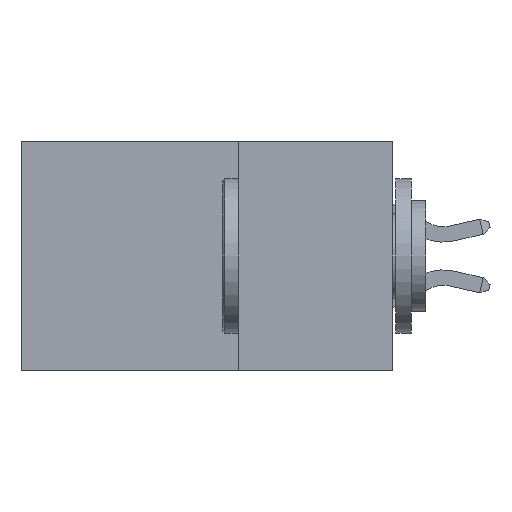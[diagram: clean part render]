
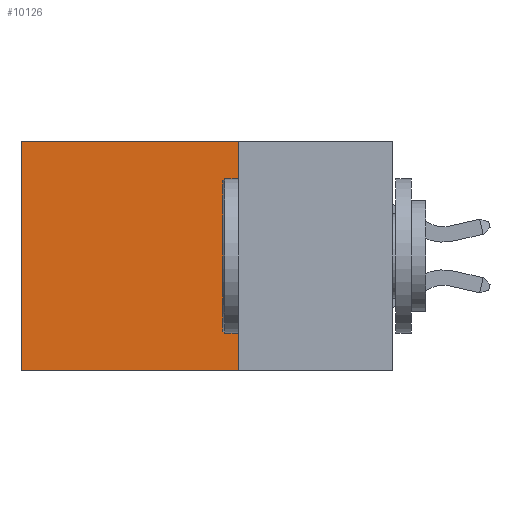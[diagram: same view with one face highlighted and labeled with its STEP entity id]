
A CAD part, left-side view. The second image highlights one B-rep face of the part: STEP entity #10126.
In plain terms, the highlighted planar face has unit normal (-1, 0, 0).
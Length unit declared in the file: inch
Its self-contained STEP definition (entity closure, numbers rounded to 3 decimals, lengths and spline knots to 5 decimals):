
#31 = VERTEX_POINT ( 'NONE', #9871 ) ;
#461 = EDGE_CURVE ( 'NONE', #31, #5469, #11803, .T. ) ;
#517 = CARTESIAN_POINT ( 'NONE',  ( 0.2875, 0.6, 0. ) ) ;
#1117 = LINE ( 'NONE', #2367, #7731 ) ;
#1857 = ORIENTED_EDGE ( 'NONE', *, *, #10371, .F. ) ;
#2362 = VECTOR ( 'NONE', #10039, 39.37008 ) ;
#2367 = CARTESIAN_POINT ( 'NONE',  ( 0.2875, 0.6, 0. ) ) ;
#2748 = ORIENTED_EDGE ( 'NONE', *, *, #461, .T. ) ;
#2933 = CARTESIAN_POINT ( 'NONE',  ( 0.2875, 0.25, -0.37 ) ) ;
#4209 = ORIENTED_EDGE ( 'NONE', *, *, #10594, .T. ) ;
#4328 = DIRECTION ( 'NONE',  ( 0., 0., -1. ) ) ;
#5469 = VERTEX_POINT ( 'NONE', #517 ) ;
#7024 = VECTOR ( 'NONE', #10593, 39.37008 ) ;
#7731 = VECTOR ( 'NONE', #4328, 39.37008 ) ;
#8003 = VERTEX_POINT ( 'NONE', #11242 ) ;
#8195 = CARTESIAN_POINT ( 'NONE',  ( 0.2875, 0.25, 0. ) ) ;
#8734 = LINE ( 'NONE', #2933, #7024 ) ;
#8857 = VECTOR ( 'NONE', #11675, 39.37008 ) ;
#9334 = CARTESIAN_POINT ( 'NONE',  ( 0.2875, 0.25, -0.37 ) ) ;
#9871 = CARTESIAN_POINT ( 'NONE',  ( 0.2875, 0.25, 0. ) ) ;
#10039 = DIRECTION ( 'NONE',  ( 0., 0., -1. ) ) ;
#10126 = ADVANCED_FACE ( 'NONE', ( #14295 ), #13744, .F. ) ;
#10128 = VERTEX_POINT ( 'NONE', #9334 ) ;
#10371 = EDGE_CURVE ( 'NONE', #31, #10128, #14280, .T. ) ;
#10593 = DIRECTION ( 'NONE',  ( 0., 1., 0. ) ) ;
#10594 = EDGE_CURVE ( 'NONE', #5469, #8003, #1117, .T. ) ;
#10637 = CARTESIAN_POINT ( 'NONE',  ( 0.2875, 0.25, 0. ) ) ;
#11242 = CARTESIAN_POINT ( 'NONE',  ( 0.2875, 0.6, -0.37 ) ) ;
#11675 = DIRECTION ( 'NONE',  ( 0., 1., 0. ) ) ;
#11730 = EDGE_CURVE ( 'NONE', #10128, #8003, #8734, .T. ) ;
#11803 = LINE ( 'NONE', #10637, #8857 ) ;
#12281 = AXIS2_PLACEMENT_3D ( 'NONE', #8195, #13981, #12867 ) ;
#12694 = ORIENTED_EDGE ( 'NONE', *, *, #11730, .F. ) ;
#12867 = DIRECTION ( 'NONE',  ( 0., 0., -1. ) ) ;
#13346 = CARTESIAN_POINT ( 'NONE',  ( 0.2875, 0.25, 0. ) ) ;
#13744 = PLANE ( 'NONE',  #12281 ) ;
#13981 = DIRECTION ( 'NONE',  ( 1., 0., 0. ) ) ;
#14280 = LINE ( 'NONE', #13346, #2362 ) ;
#14295 = FACE_OUTER_BOUND ( 'NONE', #14341, .T. ) ;
#14341 = EDGE_LOOP ( 'NONE', ( #4209, #12694, #1857, #2748 ) ) ;
